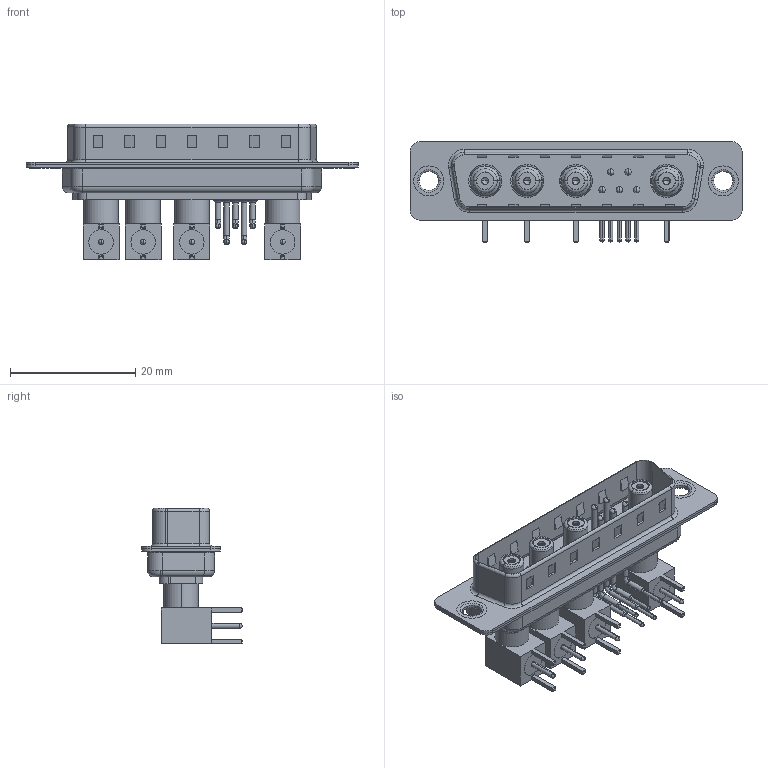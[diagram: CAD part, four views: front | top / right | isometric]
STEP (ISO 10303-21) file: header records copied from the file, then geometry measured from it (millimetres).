
FILE_DESCRIPTION (( 'STEP AP203' ), '1' );
FILE_NAME ('629-9W4-240-5N1.STEP', '2022-05-07T14:22:22', ( '' ), ( '' ), 'SwSTEP 2.0', 'SolidWorks 2020', '' );
FILE_SCHEMA (( 'CONFIG_CONTROL_DESIGN' ));
Length unit declared in the file: millimetre
Products named in the file (18): Co-Ax Jack Assy_RA; 629-9W4-240-5N1; Insulator RA Pin; Socket_RA; 629Combo Thru Hole Rivet; Insulator Socket; RA Back Shell; 629Combo Shell Rear_25 Contacts; 629Combo Contact Row 1; 629Combo Housing_9W4; Insulator Socket 2; Co-Ax Jack_RA PC Tail; 629Combo Contact Row 2; 629Combo Shell Front_25 Contacts; Locking Collar
Assembly tree (42 placements, depth 3):
  629-9W4-240-5N1
    629Combo Housing_9W4
    629Combo Shell Rear_25 Contacts
    629Combo Shell Front_25 Contacts
    629Combo Thru Hole Rivet  x2
    Co-Ax Jack Assy_RA
      Co-Ax Jack_RA PC Tail
      Insulator Socket
      Insulator Socket 2
      Locking Collar
      Socket_RA
      RA Back Shell
      Insulator RA Pin
    Co-Ax Jack Assy_RA
      Co-Ax Jack_RA PC Tail
      Insulator Socket
      Insulator Socket 2
      Locking Collar
      Socket_RA
      RA Back Shell
      Insulator RA Pin
    Co-Ax Jack Assy_RA
      Co-Ax Jack_RA PC Tail
      Insulator Socket
      Insulator Socket 2
      Locking Collar
      Socket_RA
      RA Back Shell
      Insulator RA Pin
    Co-Ax Jack Assy_RA
      Co-Ax Jack_RA PC Tail
      Insulator Socket
      Insulator Socket 2
      Locking Collar
      Socket_RA
      RA Back Shell
      Insulator RA Pin
    629Combo Contact Row 1  x2
    629Combo Contact Row 2  x3
Bounding box: 53.05 x 16 x 21.71 mm (x, y, z)
Volume: 3820.3 mm3; surface area: 10483.8 mm2
Topology: 38 solids, 38 shells, 1508 faces, 3809 edges, 2412 vertices
Faces by surface type: plane 719, cylinder 569, cone 96, torus 82, bspline 34, sphere 8
Entity records: 25477 total; most frequent: CARTESIAN_POINT 4302, DIRECTION 4081, ORIENTED_EDGE 3744, EDGE_CURVE 1872, AXIS2_PLACEMENT_3D 1465, VERTEX_POINT 1199, LINE 1151, VECTOR 1151
